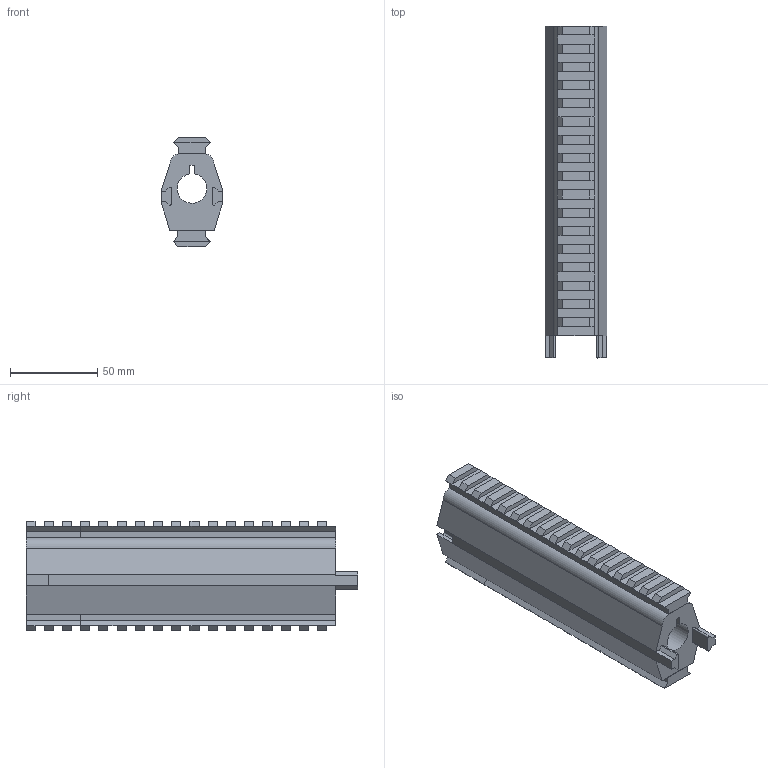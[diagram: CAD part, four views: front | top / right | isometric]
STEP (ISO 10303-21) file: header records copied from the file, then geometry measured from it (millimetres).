
FILE_DESCRIPTION(/* description */ (''),/* implementation_level */ '2;1');
FILE_NAME(/* name */ 'HRR PRA - 16in 7in Extension v4.step',/* time_stamp */ '2020-03-16T00:14:13-04:00',/* author */ (''),/* organization */ (''),/* preprocessor_version */ 'ST-DEVELOPER v18',/* originating_system */ 'Autodesk Translation Framework v8.12.0.6',/* authorisation */ '');
FILE_SCHEMA (('AUTOMOTIVE_DESIGN { 1 0 10303 214 3 1 1 }'));
Length unit declared in the file: millimetre
Products named in the file (1): HRR PRA - 16in 7in Extension
Bounding box: 35.56 x 190.5 x 62.84 mm (x, y, z)
Volume: 242063.9 mm3; surface area: 62426.8 mm2
Topology: 5 solids, 5 shells, 278 faces, 737 edges, 469 vertices
Faces by surface type: plane 267, cylinder 11
Entity records: 8400 total; most frequent: CARTESIAN_POINT 1485, ORIENTED_EDGE 1474, DIRECTION 1317, EDGE_CURVE 737, LINE 715, VECTOR 715, VERTEX_POINT 469, AXIS2_PLACEMENT_3D 301
